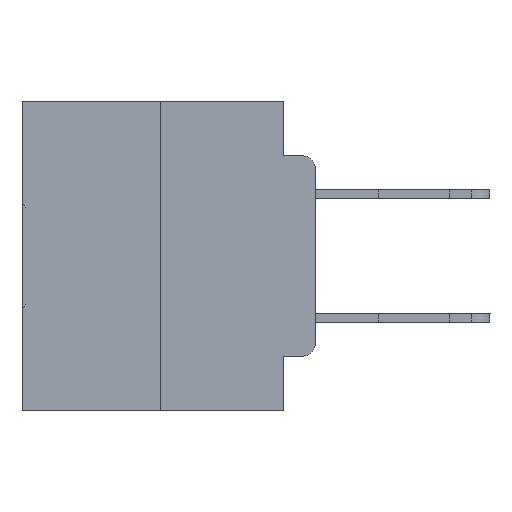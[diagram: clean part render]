
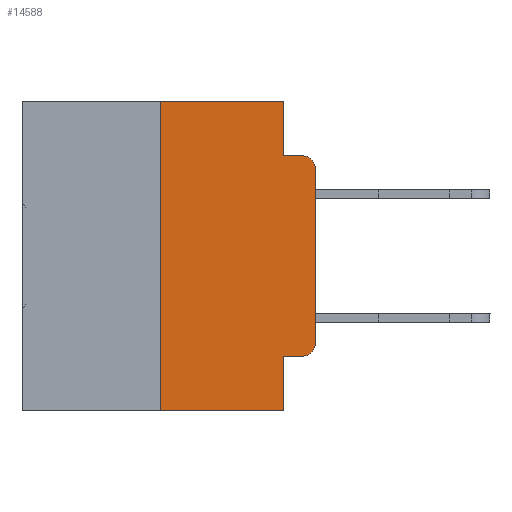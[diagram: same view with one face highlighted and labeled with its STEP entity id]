
A CAD part, left-side view. The second image highlights one B-rep face of the part: STEP entity #14588.
In plain terms, the highlighted planar face has unit normal (-1, 0, 0).
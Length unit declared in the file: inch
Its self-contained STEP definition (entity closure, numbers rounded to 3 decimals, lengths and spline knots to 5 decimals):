
#31 = ORIENTED_EDGE ( 'NONE', *, *, #13014, .F. ) ;
#159 = VERTEX_POINT ( 'NONE', #14351 ) ;
#614 = EDGE_CURVE ( 'NONE', #11899, #12149, #6027, .T. ) ;
#742 = LINE ( 'NONE', #10942, #24700 ) ;
#1346 = CARTESIAN_POINT ( 'NONE',  ( 0., 0.473, 0. ) ) ;
#1490 = DIRECTION ( 'NONE',  ( -1., 0., 0. ) ) ;
#1505 = ORIENTED_EDGE ( 'NONE', *, *, #23887, .T. ) ;
#1694 = VERTEX_POINT ( 'NONE', #28375 ) ;
#2472 = LINE ( 'NONE', #14525, #24460 ) ;
#3749 = DIRECTION ( 'NONE',  ( 0., 0., -1. ) ) ;
#3884 = ORIENTED_EDGE ( 'NONE', *, *, #26015, .T. ) ;
#3903 = CARTESIAN_POINT ( 'NONE',  ( 0., 0.051, -0.4115 ) ) ;
#3951 = CARTESIAN_POINT ( 'NONE',  ( 0., 0.473, -0.5 ) ) ;
#4439 = DIRECTION ( 'NONE',  ( -1., 0., 0. ) ) ;
#5349 = EDGE_CURVE ( 'NONE', #25051, #159, #24335, .T. ) ;
#5835 = VECTOR ( 'NONE', #11059, 39.37008 ) ;
#6027 = CIRCLE ( 'NONE', #10105, 0.02 ) ;
#6308 = DIRECTION ( 'NONE',  ( 1., 0., 0. ) ) ;
#6835 = AXIS2_PLACEMENT_3D ( 'NONE', #28908, #4439, #14116 ) ;
#6926 = VECTOR ( 'NONE', #22987, 39.37008 ) ;
#8134 = ORIENTED_EDGE ( 'NONE', *, *, #12934, .F. ) ;
#8776 = CARTESIAN_POINT ( 'NONE',  ( 0., 0.051, -0.4115 ) ) ;
#8990 = PLANE ( 'NONE',  #14400 ) ;
#9176 = VERTEX_POINT ( 'NONE', #3903 ) ;
#10105 = AXIS2_PLACEMENT_3D ( 'NONE', #26281, #1490, #23805 ) ;
#10257 = EDGE_CURVE ( 'NONE', #9176, #11899, #14783, .T. ) ;
#10942 = CARTESIAN_POINT ( 'NONE',  ( 0., 0.051, 0. ) ) ;
#11038 = ORIENTED_EDGE ( 'NONE', *, *, #27250, .F. ) ;
#11059 = DIRECTION ( 'NONE',  ( 0., -1., 0. ) ) ;
#11208 = CARTESIAN_POINT ( 'NONE',  ( 0., 0.051, -0.5 ) ) ;
#11457 = DIRECTION ( 'NONE',  ( 0., -1., 0. ) ) ;
#11509 = LINE ( 'NONE', #16739, #6926 ) ;
#11899 = VERTEX_POINT ( 'NONE', #27970 ) ;
#12149 = VERTEX_POINT ( 'NONE', #16311 ) ;
#12690 = ORIENTED_EDGE ( 'NONE', *, *, #5349, .T. ) ;
#12934 = EDGE_CURVE ( 'NONE', #9176, #31412, #30080, .T. ) ;
#13014 = EDGE_CURVE ( 'NONE', #26017, #159, #11509, .T. ) ;
#13744 = DIRECTION ( 'NONE',  ( 0., -1., 0. ) ) ;
#13964 = VERTEX_POINT ( 'NONE', #19174 ) ;
#14116 = DIRECTION ( 'NONE',  ( 0., 0., -1. ) ) ;
#14351 = CARTESIAN_POINT ( 'NONE',  ( 0., 0.02, -0.0885 ) ) ;
#14354 = CARTESIAN_POINT ( 'NONE',  ( 0., 0., -0.1085 ) ) ;
#14399 = VERTEX_POINT ( 'NONE', #28203 ) ;
#14400 = AXIS2_PLACEMENT_3D ( 'NONE', #1346, #6308, #26353 ) ;
#14525 = CARTESIAN_POINT ( 'NONE',  ( 0., 0., 0. ) ) ;
#14588 = ADVANCED_FACE ( 'NONE', ( #21991 ), #8990, .F. ) ;
#14783 = LINE ( 'NONE', #8776, #20981 ) ;
#15394 = VECTOR ( 'NONE', #27094, 39.37008 ) ;
#16311 = CARTESIAN_POINT ( 'NONE',  ( 0., 0., -0.3915 ) ) ;
#16533 = ORIENTED_EDGE ( 'NONE', *, *, #27224, .F. ) ;
#16739 = CARTESIAN_POINT ( 'NONE',  ( 0., 0.051, -0.0885 ) ) ;
#17874 = VECTOR ( 'NONE', #19573, 39.37008 ) ;
#19174 = CARTESIAN_POINT ( 'NONE',  ( 0., 0.25, 0. ) ) ;
#19250 = EDGE_CURVE ( 'NONE', #14399, #13964, #28291, .T. ) ;
#19390 = ORIENTED_EDGE ( 'NONE', *, *, #19250, .F. ) ;
#19573 = DIRECTION ( 'NONE',  ( 0., 0., 1. ) ) ;
#20981 = VECTOR ( 'NONE', #11457, 39.37008 ) ;
#21991 = FACE_OUTER_BOUND ( 'NONE', #25684, .T. ) ;
#22987 = DIRECTION ( 'NONE',  ( 0., -1., 0. ) ) ;
#23506 = LINE ( 'NONE', #30602, #25075 ) ;
#23805 = DIRECTION ( 'NONE',  ( 0., 0., -1. ) ) ;
#23887 = EDGE_CURVE ( 'NONE', #12149, #25051, #2472, .T. ) ;
#24335 = CIRCLE ( 'NONE', #6835, 0.02 ) ;
#24388 = CARTESIAN_POINT ( 'NONE',  ( 0., 0.051, 0. ) ) ;
#24460 = VECTOR ( 'NONE', #27139, 39.37008 ) ;
#24700 = VECTOR ( 'NONE', #3749, 39.37008 ) ;
#25051 = VERTEX_POINT ( 'NONE', #14354 ) ;
#25075 = VECTOR ( 'NONE', #13744, 39.37008 ) ;
#25684 = EDGE_LOOP ( 'NONE', ( #1505, #12690, #31, #16533, #11038, #19390, #3884, #8134, #29840, #27836 ) ) ;
#26015 = EDGE_CURVE ( 'NONE', #14399, #31412, #28616, .T. ) ;
#26017 = VERTEX_POINT ( 'NONE', #28632 ) ;
#26281 = CARTESIAN_POINT ( 'NONE',  ( 0., 0.02, -0.3915 ) ) ;
#26353 = DIRECTION ( 'NONE',  ( 0., 0., -1. ) ) ;
#27005 = CARTESIAN_POINT ( 'NONE',  ( 0., 0.25, 0. ) ) ;
#27094 = DIRECTION ( 'NONE',  ( 0., 0., -1. ) ) ;
#27139 = DIRECTION ( 'NONE',  ( 0., 0., 1. ) ) ;
#27224 = EDGE_CURVE ( 'NONE', #1694, #26017, #742, .T. ) ;
#27250 = EDGE_CURVE ( 'NONE', #13964, #1694, #23506, .T. ) ;
#27836 = ORIENTED_EDGE ( 'NONE', *, *, #614, .T. ) ;
#27970 = CARTESIAN_POINT ( 'NONE',  ( 0., 0.02, -0.4115 ) ) ;
#28203 = CARTESIAN_POINT ( 'NONE',  ( 0., 0.25, -0.5 ) ) ;
#28291 = LINE ( 'NONE', #27005, #17874 ) ;
#28375 = CARTESIAN_POINT ( 'NONE',  ( 0., 0.051, 0. ) ) ;
#28616 = LINE ( 'NONE', #3951, #5835 ) ;
#28632 = CARTESIAN_POINT ( 'NONE',  ( 0., 0.051, -0.0885 ) ) ;
#28908 = CARTESIAN_POINT ( 'NONE',  ( 0., 0.02, -0.1085 ) ) ;
#29840 = ORIENTED_EDGE ( 'NONE', *, *, #10257, .T. ) ;
#30080 = LINE ( 'NONE', #24388, #15394 ) ;
#30602 = CARTESIAN_POINT ( 'NONE',  ( 0., 0.473, 0. ) ) ;
#31412 = VERTEX_POINT ( 'NONE', #11208 ) ;
